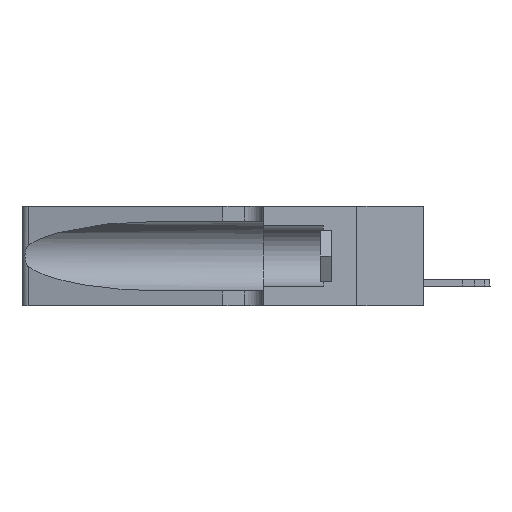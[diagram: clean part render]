
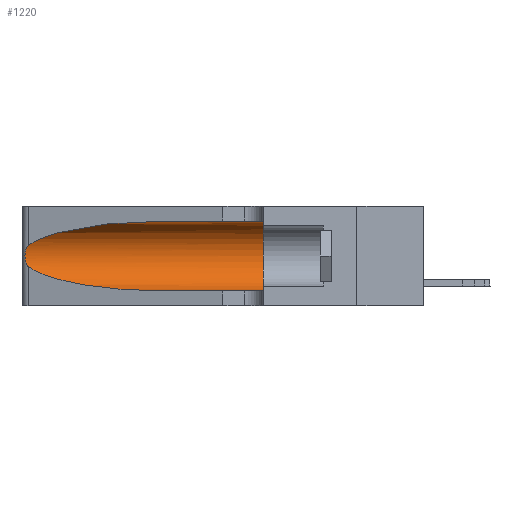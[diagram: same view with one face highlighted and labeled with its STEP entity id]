
A CAD part, left-side view. The second image highlights one B-rep face of the part: STEP entity #1220.
In plain terms, the highlighted cylindrical face has radius 3.308 mm (diameter 6.617 mm), a partial arc.
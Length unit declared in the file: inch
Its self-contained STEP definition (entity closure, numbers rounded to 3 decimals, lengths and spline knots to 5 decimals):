
#497 = CYLINDRICAL_SURFACE ( 'NONE', #11304, 0.13025 ) ;
#551 = DIRECTION ( 'NONE',  ( 0., -1., 0. ) ) ;
#856 = ORIENTED_EDGE ( 'NONE', *, *, #14074, .F. ) ;
#1105 = CARTESIAN_POINT ( 'NONE',  ( 0.25487, 1.22718, 0.14631 ) ) ;
#1220 = ADVANCED_FACE ( 'NONE', ( #12172 ), #497, .F. ) ;
#1324 = CARTESIAN_POINT ( 'NONE',  ( 0.25639, 1.23186, 0.15144 ) ) ;
#1526 = CARTESIAN_POINT ( 'NONE',  ( 0.26018, 1.23835, 0.19895 ) ) ;
#1529 = B_SPLINE_CURVE_WITH_KNOTS ( 'NONE', 3,
 ( #14677, #19349, #8610, #4041, #10656, #1526, #10722, #15394, #4478, #16933, #5991, #1324, #20117, #7664 ),
 .UNSPECIFIED., .F., .F.,
 ( 4, 2, 2, 2, 2, 2, 4 ),
 ( 0., 0.00027, 0.00053, 0.00107, 0.0016, 0.00187, 0.00214 ),
 .UNSPECIFIED. ) ;
#1553 = VERTEX_POINT ( 'NONE', #1105 ) ;
#1818 = DIRECTION ( 'NONE',  ( 0., 0., -1. ) ) ;
#1930 = CARTESIAN_POINT ( 'NONE',  ( 0.1305, 0.35, 0.31525 ) ) ;
#2147 = ORIENTED_EDGE ( 'NONE', *, *, #9253, .F. ) ;
#2326 = VERTEX_POINT ( 'NONE', #14513 ) ;
#2411 = LINE ( 'NONE', #9809, #8757 ) ;
#2554 = DIRECTION ( 'NONE',  ( 0., 1., 0. ) ) ;
#2916 = CARTESIAN_POINT ( 'NONE',  ( 0.2373, 1.15595, 0.28018 ) ) ;
#2970 = ORIENTED_EDGE ( 'NONE', *, *, #18626, .T. ) ;
#3229 = VECTOR ( 'NONE', #551, 39.37008 ) ;
#4041 = CARTESIAN_POINT ( 'NONE',  ( 0.25787, 1.23484, 0.2124 ) ) ;
#4329 = CARTESIAN_POINT ( 'NONE',  ( 0.1305, 0.35, 0.185 ) ) ;
#4478 = CARTESIAN_POINT ( 'NONE',  ( 0.26017, 1.23833, 0.17102 ) ) ;
#4664 = VERTEX_POINT ( 'NONE', #8897 ) ;
#5440 = AXIS2_PLACEMENT_3D ( 'NONE', #4329, #2554, #5758 ) ;
#5758 = DIRECTION ( 'NONE',  ( 0., 0., 1. ) ) ;
#5991 = CARTESIAN_POINT ( 'NONE',  ( 0.25789, 1.23486, 0.15765 ) ) ;
#6060 =( BOUNDED_CURVE ( )  B_SPLINE_CURVE ( 3, ( #18942, #17433, #18662, #9417 ),
 .UNSPECIFIED., .F., .F. ) 
 B_SPLINE_CURVE_WITH_KNOTS ( ( 4, 4 ),
 ( 3.44316, 4.71239 ),
 .UNSPECIFIED. ) 
 CURVE ( )  GEOMETRIC_REPRESENTATION_ITEM ( )  RATIONAL_B_SPLINE_CURVE ( ( 1., 0.87, 0.87, 1. ) ) 
 REPRESENTATION_ITEM ( '' )  );
#6818 = ORIENTED_EDGE ( 'NONE', *, *, #17288, .T. ) ;
#7664 = CARTESIAN_POINT ( 'NONE',  ( 0.25487, 1.22718, 0.14631 ) ) ;
#7685 = CARTESIAN_POINT ( 'NONE',  ( 0.25487, 1.22718, 0.22369 ) ) ;
#8024 = VERTEX_POINT ( 'NONE', #1930 ) ;
#8237 = CARTESIAN_POINT ( 'NONE',  ( 0.1305, 0.72297, 0.31525 ) ) ;
#8408 = CARTESIAN_POINT ( 'NONE',  ( 0.1305, 0.35, 0.05475 ) ) ;
#8610 = CARTESIAN_POINT ( 'NONE',  ( 0.25639, 1.23184, 0.21858 ) ) ;
#8757 = VECTOR ( 'NONE', #19530, 39.37008 ) ;
#8897 = CARTESIAN_POINT ( 'NONE',  ( 0.25487, 1.22718, 0.22369 ) ) ;
#9253 = EDGE_CURVE ( 'NONE', #8024, #18940, #10603, .T. ) ;
#9417 = CARTESIAN_POINT ( 'NONE',  ( 0.1305, 0.72297, 0.05475 ) ) ;
#9660 =( BOUNDED_CURVE ( )  B_SPLINE_CURVE ( 3, ( #13684, #12197, #2916, #7685 ),
 .UNSPECIFIED., .F., .T. ) 
 B_SPLINE_CURVE_WITH_KNOTS ( ( 4, 4 ),
 ( 1.5708, 2.84003 ),
 .UNSPECIFIED. ) 
 CURVE ( )  GEOMETRIC_REPRESENTATION_ITEM ( )  RATIONAL_B_SPLINE_CURVE ( ( 1., 0.87, 0.87, 1. ) ) 
 REPRESENTATION_ITEM ( '' )  );
#9780 = EDGE_CURVE ( 'NONE', #15307, #4664, #9660, .T. ) ;
#9809 = CARTESIAN_POINT ( 'NONE',  ( 0.1305, 1.61858, 0.31525 ) ) ;
#9904 = CARTESIAN_POINT ( 'NONE',  ( 0.1305, 1.61858, 0.05475 ) ) ;
#10603 = CIRCLE ( 'NONE', #5440, 0.13025 ) ;
#10656 = CARTESIAN_POINT ( 'NONE',  ( 0.25854, 1.2359, 0.20912 ) ) ;
#10722 = CARTESIAN_POINT ( 'NONE',  ( 0.26075, 1.23896, 0.19203 ) ) ;
#11304 = AXIS2_PLACEMENT_3D ( 'NONE', #18970, #15595, #1818 ) ;
#12172 = FACE_OUTER_BOUND ( 'NONE', #14955, .T. ) ;
#12181 = ORIENTED_EDGE ( 'NONE', *, *, #17408, .T. ) ;
#12197 = CARTESIAN_POINT ( 'NONE',  ( 0.18966, 0.96281, 0.31525 ) ) ;
#13375 = ORIENTED_EDGE ( 'NONE', *, *, #9780, .T. ) ;
#13684 = CARTESIAN_POINT ( 'NONE',  ( 0.1305, 0.72297, 0.31525 ) ) ;
#14074 = EDGE_CURVE ( 'NONE', #15307, #8024, #2411, .T. ) ;
#14163 = LINE ( 'NONE', #9904, #3229 ) ;
#14513 = CARTESIAN_POINT ( 'NONE',  ( 0.1305, 0.72297, 0.05475 ) ) ;
#14677 = CARTESIAN_POINT ( 'NONE',  ( 0.25487, 1.22718, 0.22369 ) ) ;
#14955 = EDGE_LOOP ( 'NONE', ( #13375, #12181, #6818, #2970, #2147, #856 ) ) ;
#15307 = VERTEX_POINT ( 'NONE', #8237 ) ;
#15394 = CARTESIAN_POINT ( 'NONE',  ( 0.26075, 1.23896, 0.178 ) ) ;
#15595 = DIRECTION ( 'NONE',  ( 0., -1., 0. ) ) ;
#16933 = CARTESIAN_POINT ( 'NONE',  ( 0.25856, 1.23593, 0.16098 ) ) ;
#17288 = EDGE_CURVE ( 'NONE', #1553, #2326, #6060, .T. ) ;
#17408 = EDGE_CURVE ( 'NONE', #4664, #1553, #1529, .T. ) ;
#17433 = CARTESIAN_POINT ( 'NONE',  ( 0.2373, 1.15595, 0.08982 ) ) ;
#18626 = EDGE_CURVE ( 'NONE', #2326, #18940, #14163, .T. ) ;
#18662 = CARTESIAN_POINT ( 'NONE',  ( 0.18966, 0.96281, 0.05475 ) ) ;
#18940 = VERTEX_POINT ( 'NONE', #8408 ) ;
#18942 = CARTESIAN_POINT ( 'NONE',  ( 0.25487, 1.22718, 0.14631 ) ) ;
#18970 = CARTESIAN_POINT ( 'NONE',  ( 0.1305, 1.61858, 0.185 ) ) ;
#19349 = CARTESIAN_POINT ( 'NONE',  ( 0.25555, 1.22994, 0.2215 ) ) ;
#19530 = DIRECTION ( 'NONE',  ( 0., -1., 0. ) ) ;
#20117 = CARTESIAN_POINT ( 'NONE',  ( 0.25555, 1.22993, 0.14849 ) ) ;
